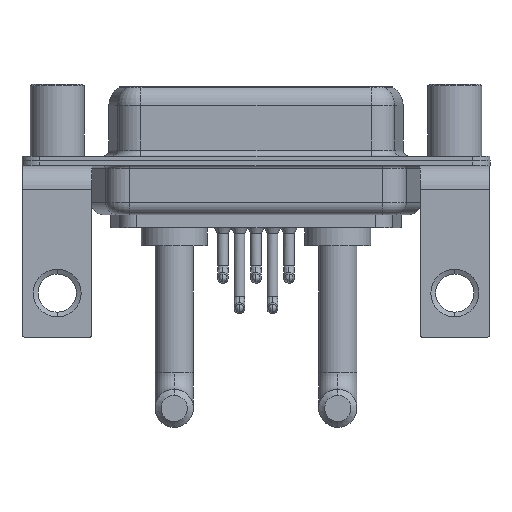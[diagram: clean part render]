
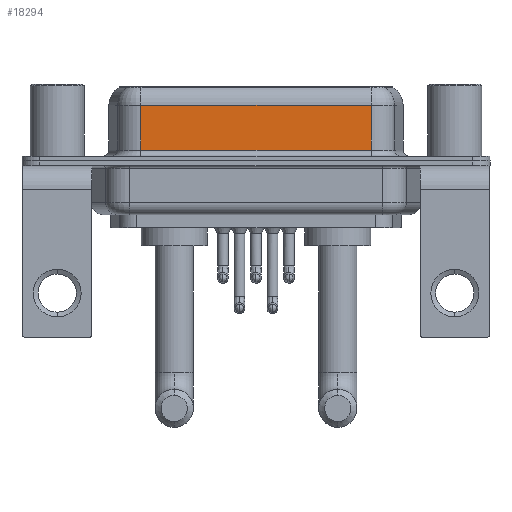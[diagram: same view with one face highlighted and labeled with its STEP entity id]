
A CAD part, front view. The second image highlights one B-rep face of the part: STEP entity #18294.
In plain terms, the highlighted planar face has unit normal (0, -1, 0).
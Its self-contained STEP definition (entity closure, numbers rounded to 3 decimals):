
#451 = DIRECTION ( 'NONE',  ( 1., 0., 0. ) ) ;
#646 = CARTESIAN_POINT ( 'NONE',  ( 26.287, -3.95, 6.4 ) ) ;
#1021 = LINE ( 'NONE', #10114, #6808 ) ;
#2072 = DIRECTION ( 'NONE',  ( -1., 0., 0. ) ) ;
#2191 = EDGE_CURVE ( 'NONE', #14590, #8444, #3366, .T. ) ;
#2200 = CARTESIAN_POINT ( 'NONE',  ( 26.287, -3.95, 0.9 ) ) ;
#2695 = DIRECTION ( 'NONE',  ( 0., 0., -1. ) ) ;
#2922 = ORIENTED_EDGE ( 'NONE', *, *, #11821, .T. ) ;
#3366 = LINE ( 'NONE', #15516, #10708 ) ;
#3782 = FACE_OUTER_BOUND ( 'NONE', #6590, .T. ) ;
#4571 = VERTEX_POINT ( 'NONE', #4738 ) ;
#4738 = CARTESIAN_POINT ( 'NONE',  ( 7.013, -3.95, 0.9 ) ) ;
#5810 = ORIENTED_EDGE ( 'NONE', *, *, #7631, .T. ) ;
#6095 = EDGE_CURVE ( 'NONE', #14590, #15687, #7194, .T. ) ;
#6542 = DIRECTION ( 'NONE',  ( 0., 1., 0. ) ) ;
#6590 = EDGE_LOOP ( 'NONE', ( #6730, #16015, #2922, #5810 ) ) ;
#6730 = ORIENTED_EDGE ( 'NONE', *, *, #6095, .F. ) ;
#6808 = VECTOR ( 'NONE', #2695, 1000. ) ;
#6846 = DIRECTION ( 'NONE',  ( 0., 0., 1. ) ) ;
#7099 = DIRECTION ( 'NONE',  ( 0., 0., -1. ) ) ;
#7194 = LINE ( 'NONE', #13268, #16070 ) ;
#7631 = EDGE_CURVE ( 'NONE', #4571, #15687, #11123, .T. ) ;
#8444 = VERTEX_POINT ( 'NONE', #11787 ) ;
#8896 = AXIS2_PLACEMENT_3D ( 'NONE', #646, #6542, #6846 ) ;
#10114 = CARTESIAN_POINT ( 'NONE',  ( 7.013, -3.95, 6.4 ) ) ;
#10708 = VECTOR ( 'NONE', #2072, 1000. ) ;
#11123 = LINE ( 'NONE', #2200, #19269 ) ;
#11787 = CARTESIAN_POINT ( 'NONE',  ( 7.013, -3.95, 4.65 ) ) ;
#11821 = EDGE_CURVE ( 'NONE', #8444, #4571, #1021, .T. ) ;
#13268 = CARTESIAN_POINT ( 'NONE',  ( 26.287, -3.95, 6.4 ) ) ;
#13848 = CARTESIAN_POINT ( 'NONE',  ( 26.287, -3.95, 4.65 ) ) ;
#14590 = VERTEX_POINT ( 'NONE', #13848 ) ;
#15516 = CARTESIAN_POINT ( 'NONE',  ( 26.287, -3.95, 4.65 ) ) ;
#15687 = VERTEX_POINT ( 'NONE', #17658 ) ;
#16015 = ORIENTED_EDGE ( 'NONE', *, *, #2191, .T. ) ;
#16070 = VECTOR ( 'NONE', #7099, 1000. ) ;
#17152 = PLANE ( 'NONE',  #8896 ) ;
#17658 = CARTESIAN_POINT ( 'NONE',  ( 26.287, -3.95, 0.9 ) ) ;
#18294 = ADVANCED_FACE ( 'NONE', ( #3782 ), #17152, .F. ) ;
#19269 = VECTOR ( 'NONE', #451, 1000. ) ;
